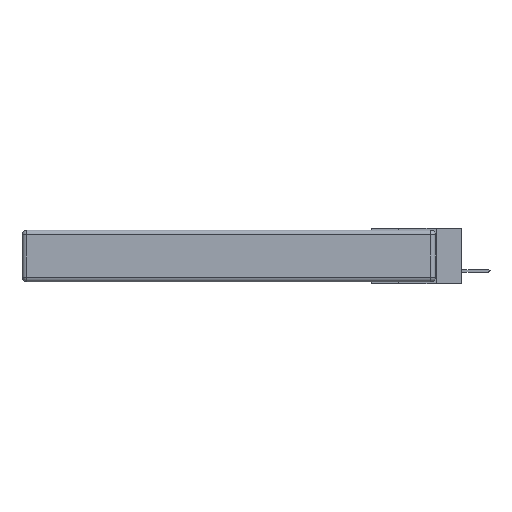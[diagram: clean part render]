
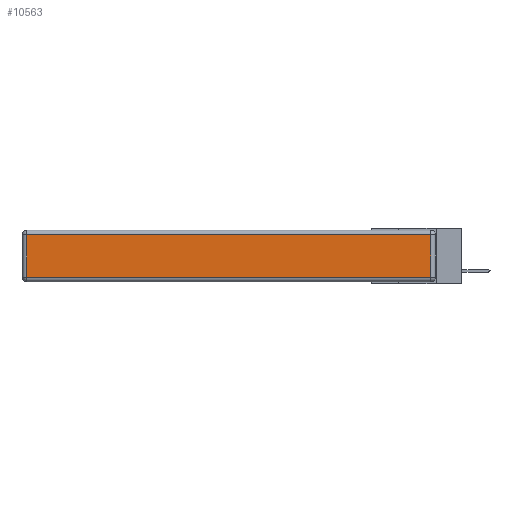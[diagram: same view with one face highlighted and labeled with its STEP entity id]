
A CAD part, left-side view. The second image highlights one B-rep face of the part: STEP entity #10563.
In plain terms, the highlighted planar face has unit normal (-1, 0, 0).
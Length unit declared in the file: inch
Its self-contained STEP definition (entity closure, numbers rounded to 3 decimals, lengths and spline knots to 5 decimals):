
#113 = VECTOR ( 'NONE', #11338, 39.37008 ) ;
#334 = LINE ( 'NONE', #11256, #10783 ) ;
#560 = ORIENTED_EDGE ( 'NONE', *, *, #11666, .T. ) ;
#1123 = CARTESIAN_POINT ( 'NONE',  ( 0., 2.72, -0.343 ) ) ;
#1570 = LINE ( 'NONE', #1123, #113 ) ;
#2003 = DIRECTION ( 'NONE',  ( 0., 1., 0. ) ) ;
#2704 = VERTEX_POINT ( 'NONE', #11885 ) ;
#3747 = PLANE ( 'NONE',  #4652 ) ;
#4065 = ORIENTED_EDGE ( 'NONE', *, *, #12909, .T. ) ;
#4208 = EDGE_LOOP ( 'NONE', ( #7442, #6408, #560, #4065 ) ) ;
#4210 = EDGE_CURVE ( 'NONE', #9678, #2704, #12948, .T. ) ;
#4652 = AXIS2_PLACEMENT_3D ( 'NONE', #11917, #8786, #9868 ) ;
#5173 = FACE_OUTER_BOUND ( 'NONE', #4208, .T. ) ;
#6204 = CARTESIAN_POINT ( 'NONE',  ( 0., 0., -0.313 ) ) ;
#6291 = DIRECTION ( 'NONE',  ( 0., -1., 0. ) ) ;
#6408 = ORIENTED_EDGE ( 'NONE', *, *, #7203, .T. ) ;
#7203 = EDGE_CURVE ( 'NONE', #2704, #7678, #8610, .T. ) ;
#7442 = ORIENTED_EDGE ( 'NONE', *, *, #4210, .T. ) ;
#7678 = VERTEX_POINT ( 'NONE', #9608 ) ;
#8408 = VERTEX_POINT ( 'NONE', #12649 ) ;
#8610 = LINE ( 'NONE', #9274, #10915 ) ;
#8786 = DIRECTION ( 'NONE',  ( -1., 0., 0. ) ) ;
#9274 = CARTESIAN_POINT ( 'NONE',  ( 0., 0.03, -0.343 ) ) ;
#9324 = DIRECTION ( 'NONE',  ( 0., 0., 1. ) ) ;
#9608 = CARTESIAN_POINT ( 'NONE',  ( 0., 0.03, -0.03 ) ) ;
#9678 = VERTEX_POINT ( 'NONE', #9878 ) ;
#9868 = DIRECTION ( 'NONE',  ( 0., 0., 1. ) ) ;
#9878 = CARTESIAN_POINT ( 'NONE',  ( 0., 2.72, -0.313 ) ) ;
#10189 = VECTOR ( 'NONE', #6291, 39.37008 ) ;
#10563 = ADVANCED_FACE ( 'NONE', ( #5173 ), #3747, .T. ) ;
#10783 = VECTOR ( 'NONE', #2003, 39.37008 ) ;
#10915 = VECTOR ( 'NONE', #9324, 39.37008 ) ;
#11256 = CARTESIAN_POINT ( 'NONE',  ( 0., 2.75, -0.03 ) ) ;
#11338 = DIRECTION ( 'NONE',  ( 0., 0., -1. ) ) ;
#11666 = EDGE_CURVE ( 'NONE', #7678, #8408, #334, .T. ) ;
#11885 = CARTESIAN_POINT ( 'NONE',  ( 0., 0.03, -0.313 ) ) ;
#11917 = CARTESIAN_POINT ( 'NONE',  ( 0., 0., -0.343 ) ) ;
#12649 = CARTESIAN_POINT ( 'NONE',  ( 0., 2.72, -0.03 ) ) ;
#12909 = EDGE_CURVE ( 'NONE', #8408, #9678, #1570, .T. ) ;
#12948 = LINE ( 'NONE', #6204, #10189 ) ;
